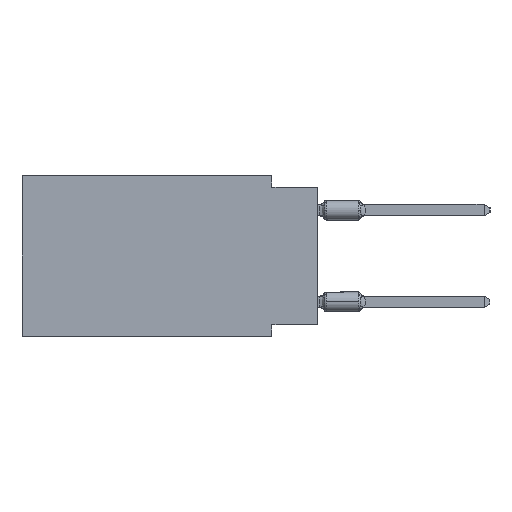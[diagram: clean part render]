
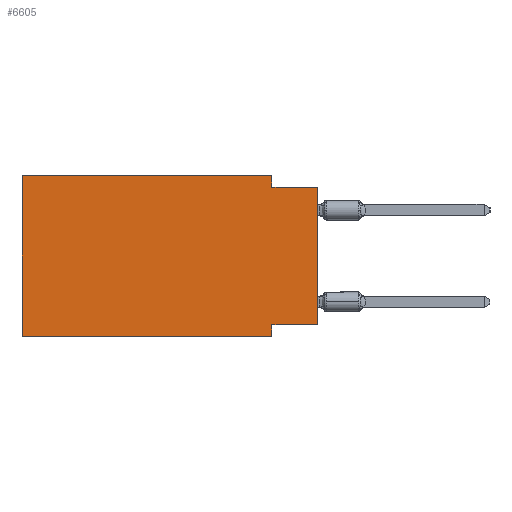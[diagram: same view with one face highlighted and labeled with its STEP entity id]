
A CAD part, left-side view. The second image highlights one B-rep face of the part: STEP entity #6605.
In plain terms, the highlighted planar face has unit normal (-1, 0, 0).
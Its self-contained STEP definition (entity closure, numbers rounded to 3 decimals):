
#764 = DIRECTION ( 'NONE',  ( 1., 0., 0. ) ) ;
#1092 = VERTEX_POINT ( 'NONE', #20409 ) ;
#1232 = ORIENTED_EDGE ( 'NONE', *, *, #44049, .F. ) ;
#1784 = ORIENTED_EDGE ( 'NONE', *, *, #9858, .F. ) ;
#3095 = DIRECTION ( 'NONE',  ( 0., 1., 0. ) ) ;
#3233 = ORIENTED_EDGE ( 'NONE', *, *, #51387, .T. ) ;
#3505 = CARTESIAN_POINT ( 'NONE',  ( 0., 16.383, 0. ) ) ;
#4139 = LINE ( 'NONE', #41462, #8690 ) ;
#5052 = DIRECTION ( 'NONE',  ( 0., 0., 1. ) ) ;
#5609 = LINE ( 'NONE', #8830, #38563 ) ;
#5827 = VERTEX_POINT ( 'NONE', #41729 ) ;
#6420 = ORIENTED_EDGE ( 'NONE', *, *, #27323, .F. ) ;
#6605 = ADVANCED_FACE ( 'NONE', ( #38091 ), #17693, .F. ) ;
#8020 = ORIENTED_EDGE ( 'NONE', *, *, #19234, .F. ) ;
#8466 = CARTESIAN_POINT ( 'NONE',  ( 0., 2.54, -8.89 ) ) ;
#8654 = VERTEX_POINT ( 'NONE', #28599 ) ;
#8690 = VECTOR ( 'NONE', #37683, 1000. ) ;
#8830 = CARTESIAN_POINT ( 'NONE',  ( 0., 0., 0. ) ) ;
#9858 = EDGE_CURVE ( 'NONE', #8654, #32082, #32902, .T. ) ;
#12409 = LINE ( 'NONE', #44363, #37875 ) ;
#12677 = EDGE_CURVE ( 'NONE', #1092, #43933, #14634, .T. ) ;
#14634 = LINE ( 'NONE', #31031, #26415 ) ;
#17334 = VECTOR ( 'NONE', #39449, 1000. ) ;
#17693 = PLANE ( 'NONE',  #25229 ) ;
#18469 = VERTEX_POINT ( 'NONE', #46320 ) ;
#19234 = EDGE_CURVE ( 'NONE', #18469, #52020, #24460, .T. ) ;
#20409 = CARTESIAN_POINT ( 'NONE',  ( 0., 0., -8.255 ) ) ;
#23678 = DIRECTION ( 'NONE',  ( 0., -1., 0. ) ) ;
#24460 = LINE ( 'NONE', #3505, #49165 ) ;
#25229 = AXIS2_PLACEMENT_3D ( 'NONE', #34328, #764, #34067 ) ;
#26350 = LINE ( 'NONE', #27375, #17334 ) ;
#26415 = VECTOR ( 'NONE', #3095, 1000. ) ;
#26691 = EDGE_LOOP ( 'NONE', ( #40159, #1784, #40898, #1232, #8020, #3233, #6420, #35247 ) ) ;
#27323 = EDGE_CURVE ( 'NONE', #43933, #5827, #36914, .T. ) ;
#27375 = CARTESIAN_POINT ( 'NONE',  ( 0., 2.54, 0. ) ) ;
#28599 = CARTESIAN_POINT ( 'NONE',  ( 0., 2.54, -0.635 ) ) ;
#31031 = CARTESIAN_POINT ( 'NONE',  ( 0., 0., -8.255 ) ) ;
#31807 = CARTESIAN_POINT ( 'NONE',  ( 0., 2.54, -8.255 ) ) ;
#32082 = VERTEX_POINT ( 'NONE', #37397 ) ;
#32902 = LINE ( 'NONE', #45261, #43470 ) ;
#33362 = VERTEX_POINT ( 'NONE', #37038 ) ;
#33529 = CARTESIAN_POINT ( 'NONE',  ( 0., 16.383, 0. ) ) ;
#34067 = DIRECTION ( 'NONE',  ( 0., 0., -1. ) ) ;
#34328 = CARTESIAN_POINT ( 'NONE',  ( 0., 16.383, 0. ) ) ;
#35247 = ORIENTED_EDGE ( 'NONE', *, *, #12677, .F. ) ;
#35812 = EDGE_CURVE ( 'NONE', #1092, #32082, #5609, .T. ) ;
#36914 = LINE ( 'NONE', #8466, #47337 ) ;
#37038 = CARTESIAN_POINT ( 'NONE',  ( 0., 2.54, 0. ) ) ;
#37397 = CARTESIAN_POINT ( 'NONE',  ( 0., 0., -0.635 ) ) ;
#37683 = DIRECTION ( 'NONE',  ( 0., -1., 0. ) ) ;
#37875 = VECTOR ( 'NONE', #23678, 1000. ) ;
#38091 = FACE_OUTER_BOUND ( 'NONE', #26691, .T. ) ;
#38563 = VECTOR ( 'NONE', #5052, 1000. ) ;
#39449 = DIRECTION ( 'NONE',  ( 0., 0., -1. ) ) ;
#40159 = ORIENTED_EDGE ( 'NONE', *, *, #35812, .T. ) ;
#40841 = DIRECTION ( 'NONE',  ( 0., 0., 1. ) ) ;
#40898 = ORIENTED_EDGE ( 'NONE', *, *, #50548, .F. ) ;
#41220 = DIRECTION ( 'NONE',  ( 0., 0., -1. ) ) ;
#41462 = CARTESIAN_POINT ( 'NONE',  ( 0., 16.383, 0. ) ) ;
#41729 = CARTESIAN_POINT ( 'NONE',  ( 0., 2.54, -8.89 ) ) ;
#43470 = VECTOR ( 'NONE', #45005, 1000. ) ;
#43933 = VERTEX_POINT ( 'NONE', #31807 ) ;
#44049 = EDGE_CURVE ( 'NONE', #52020, #33362, #4139, .T. ) ;
#44363 = CARTESIAN_POINT ( 'NONE',  ( 0., 16.383, -8.89 ) ) ;
#45005 = DIRECTION ( 'NONE',  ( 0., -1., 0. ) ) ;
#45261 = CARTESIAN_POINT ( 'NONE',  ( 0., 0., -0.635 ) ) ;
#46320 = CARTESIAN_POINT ( 'NONE',  ( 0., 16.383, -8.89 ) ) ;
#47337 = VECTOR ( 'NONE', #41220, 1000. ) ;
#49165 = VECTOR ( 'NONE', #40841, 1000. ) ;
#50548 = EDGE_CURVE ( 'NONE', #33362, #8654, #26350, .T. ) ;
#51387 = EDGE_CURVE ( 'NONE', #18469, #5827, #12409, .T. ) ;
#52020 = VERTEX_POINT ( 'NONE', #33529 ) ;
